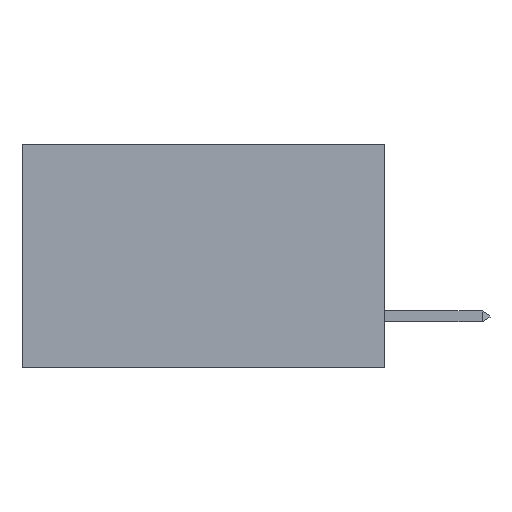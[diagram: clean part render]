
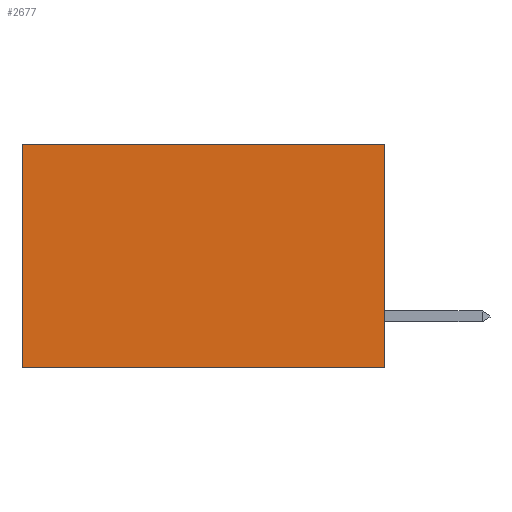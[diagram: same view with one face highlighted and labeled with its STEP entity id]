
A CAD part, left-side view. The second image highlights one B-rep face of the part: STEP entity #2677.
In plain terms, the highlighted planar face has unit normal (-1, 0, 0).
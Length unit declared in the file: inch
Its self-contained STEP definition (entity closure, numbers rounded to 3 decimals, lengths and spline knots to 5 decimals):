
#640 = ORIENTED_EDGE ( 'NONE', *, *, #12836, .F. ) ;
#641 = EDGE_LOOP ( 'NONE', ( #13539, #7209, #640, #11996 ) ) ;
#1362 = VECTOR ( 'NONE', #3050, 39.37008 ) ;
#1645 = LINE ( 'NONE', #25007, #22392 ) ;
#2677 = ADVANCED_FACE ( 'NONE', ( #24882 ), #4925, .F. ) ;
#2903 = DIRECTION ( 'NONE',  ( 0., 0., -1. ) ) ;
#3050 = DIRECTION ( 'NONE',  ( 0., 1., 0. ) ) ;
#4069 = CARTESIAN_POINT ( 'NONE',  ( 0.2875, 0., 0. ) ) ;
#4925 = PLANE ( 'NONE',  #18880 ) ;
#7209 = ORIENTED_EDGE ( 'NONE', *, *, #11647, .F. ) ;
#8071 = CARTESIAN_POINT ( 'NONE',  ( 0.2875, 0.6, -0.37 ) ) ;
#8584 = CARTESIAN_POINT ( 'NONE',  ( 0.2875, 0.6, 0. ) ) ;
#8974 = VECTOR ( 'NONE', #11747, 39.37008 ) ;
#11647 = EDGE_CURVE ( 'NONE', #22357, #18306, #12120, .T. ) ;
#11747 = DIRECTION ( 'NONE',  ( 0., 1., 0. ) ) ;
#11996 = ORIENTED_EDGE ( 'NONE', *, *, #18191, .T. ) ;
#12120 = LINE ( 'NONE', #15071, #1362 ) ;
#12836 = EDGE_CURVE ( 'NONE', #23345, #22357, #19901, .T. ) ;
#13059 = CARTESIAN_POINT ( 'NONE',  ( 0.2875, 0., -0.37 ) ) ;
#13539 = ORIENTED_EDGE ( 'NONE', *, *, #18695, .T. ) ;
#13716 = LINE ( 'NONE', #21724, #8974 ) ;
#14297 = DIRECTION ( 'NONE',  ( 0., 0., -1. ) ) ;
#15071 = CARTESIAN_POINT ( 'NONE',  ( 0.2875, 0., -0.37 ) ) ;
#17025 = DIRECTION ( 'NONE',  ( 1., 0., 0. ) ) ;
#18191 = EDGE_CURVE ( 'NONE', #23345, #23466, #13716, .T. ) ;
#18306 = VERTEX_POINT ( 'NONE', #8071 ) ;
#18695 = EDGE_CURVE ( 'NONE', #23466, #18306, #1645, .T. ) ;
#18880 = AXIS2_PLACEMENT_3D ( 'NONE', #19038, #17025, #2903 ) ;
#19038 = CARTESIAN_POINT ( 'NONE',  ( 0.2875, 0., 0. ) ) ;
#19901 = LINE ( 'NONE', #22203, #24468 ) ;
#21724 = CARTESIAN_POINT ( 'NONE',  ( 0.2875, 0., 0. ) ) ;
#22203 = CARTESIAN_POINT ( 'NONE',  ( 0.2875, 0., 0. ) ) ;
#22357 = VERTEX_POINT ( 'NONE', #13059 ) ;
#22392 = VECTOR ( 'NONE', #25086, 39.37008 ) ;
#23345 = VERTEX_POINT ( 'NONE', #4069 ) ;
#23466 = VERTEX_POINT ( 'NONE', #8584 ) ;
#24468 = VECTOR ( 'NONE', #14297, 39.37008 ) ;
#24882 = FACE_OUTER_BOUND ( 'NONE', #641, .T. ) ;
#25007 = CARTESIAN_POINT ( 'NONE',  ( 0.2875, 0.6, 0. ) ) ;
#25086 = DIRECTION ( 'NONE',  ( 0., 0., -1. ) ) ;
